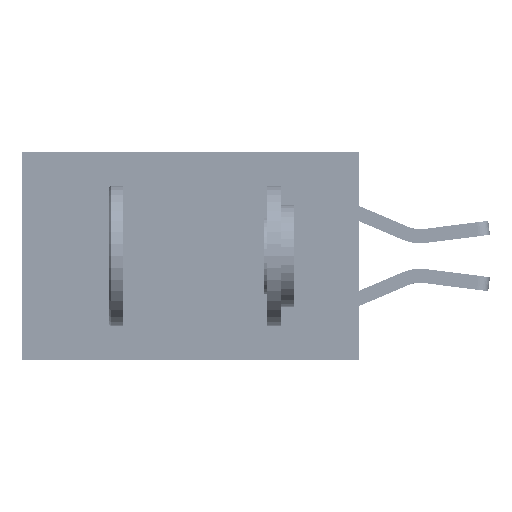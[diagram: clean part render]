
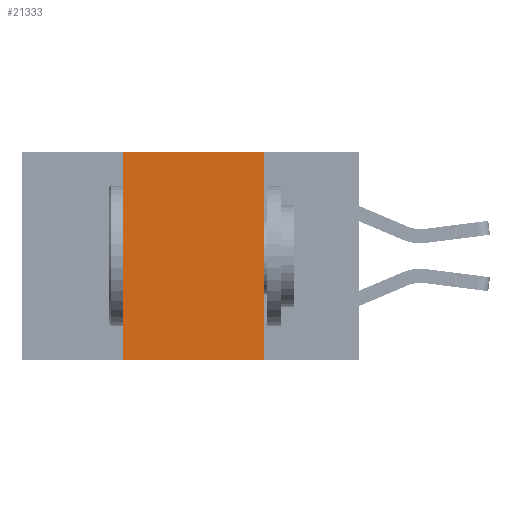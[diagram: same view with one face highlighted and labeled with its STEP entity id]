
A CAD part, left-side view. The second image highlights one B-rep face of the part: STEP entity #21333.
In plain terms, the highlighted planar face has unit normal (-1, 0, 0).
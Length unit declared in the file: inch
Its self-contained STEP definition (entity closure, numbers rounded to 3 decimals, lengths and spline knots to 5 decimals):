
#1162 = LINE ( 'NONE', #3721, #28176 ) ;
#1439 = CARTESIAN_POINT ( 'NONE',  ( 0., 0.42, 0. ) ) ;
#1935 = PLANE ( 'NONE',  #14033 ) ;
#3422 = DIRECTION ( 'NONE',  ( 0., -1., 0. ) ) ;
#3721 = CARTESIAN_POINT ( 'NONE',  ( 0., 0.6, -0.37 ) ) ;
#4631 = VECTOR ( 'NONE', #28246, 39.37008 ) ;
#5233 = CARTESIAN_POINT ( 'NONE',  ( 0., 0.42, 0. ) ) ;
#9249 = VERTEX_POINT ( 'NONE', #1439 ) ;
#10297 = DIRECTION ( 'NONE',  ( 0., -1., 0. ) ) ;
#10347 = EDGE_CURVE ( 'NONE', #17866, #24287, #18884, .T. ) ;
#10444 = CARTESIAN_POINT ( 'NONE',  ( 0., 0.17, 0. ) ) ;
#12256 = DIRECTION ( 'NONE',  ( 0., 0., -1. ) ) ;
#12680 = EDGE_CURVE ( 'NONE', #9249, #17866, #40896, .T. ) ;
#12717 = LINE ( 'NONE', #5233, #40288 ) ;
#13737 = CARTESIAN_POINT ( 'NONE',  ( 0., 0.42, -0.37 ) ) ;
#14033 = AXIS2_PLACEMENT_3D ( 'NONE', #18962, #42488, #12256 ) ;
#15241 = DIRECTION ( 'NONE',  ( 0., 0., 1. ) ) ;
#16563 = VECTOR ( 'NONE', #10297, 39.37008 ) ;
#17866 = VERTEX_POINT ( 'NONE', #10444 ) ;
#18395 = ORIENTED_EDGE ( 'NONE', *, *, #39530, .F. ) ;
#18884 = LINE ( 'NONE', #25425, #4631 ) ;
#18962 = CARTESIAN_POINT ( 'NONE',  ( 0., 0.6, 0. ) ) ;
#19672 = VERTEX_POINT ( 'NONE', #13737 ) ;
#19682 = EDGE_CURVE ( 'NONE', #19672, #24287, #1162, .T. ) ;
#21233 = EDGE_LOOP ( 'NONE', ( #36128, #42886, #18395, #30510 ) ) ;
#21333 = ADVANCED_FACE ( 'NONE', ( #27351 ), #1935, .F. ) ;
#24287 = VERTEX_POINT ( 'NONE', #24678 ) ;
#24678 = CARTESIAN_POINT ( 'NONE',  ( 0., 0.17, -0.37 ) ) ;
#25425 = CARTESIAN_POINT ( 'NONE',  ( 0., 0.17, 0. ) ) ;
#27351 = FACE_OUTER_BOUND ( 'NONE', #21233, .T. ) ;
#28176 = VECTOR ( 'NONE', #3422, 39.37008 ) ;
#28246 = DIRECTION ( 'NONE',  ( 0., 0., -1. ) ) ;
#30510 = ORIENTED_EDGE ( 'NONE', *, *, #19682, .T. ) ;
#36128 = ORIENTED_EDGE ( 'NONE', *, *, #10347, .F. ) ;
#39530 = EDGE_CURVE ( 'NONE', #19672, #9249, #12717, .T. ) ;
#40288 = VECTOR ( 'NONE', #15241, 39.37008 ) ;
#40896 = LINE ( 'NONE', #40956, #16563 ) ;
#40956 = CARTESIAN_POINT ( 'NONE',  ( 0., 0.6, 0. ) ) ;
#42488 = DIRECTION ( 'NONE',  ( 1., 0., 0. ) ) ;
#42886 = ORIENTED_EDGE ( 'NONE', *, *, #12680, .F. ) ;
